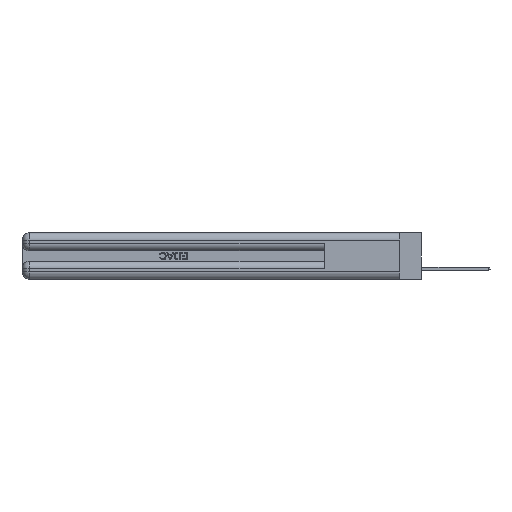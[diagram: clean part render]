
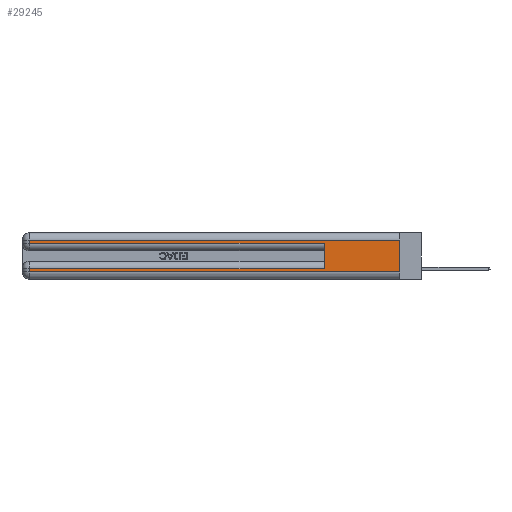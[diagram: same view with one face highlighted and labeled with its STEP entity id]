
A CAD part, left-side view. The second image highlights one B-rep face of the part: STEP entity #29245.
In plain terms, the highlighted planar face has unit normal (-1, 0, 0).
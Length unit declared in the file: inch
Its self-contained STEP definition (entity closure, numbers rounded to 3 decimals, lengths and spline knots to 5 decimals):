
#1138 = VECTOR ( 'NONE', #40566, 39.37008 ) ;
#1609 = CARTESIAN_POINT ( 'NONE',  ( 0., 0., 0.31 ) ) ;
#1885 = ORIENTED_EDGE ( 'NONE', *, *, #44636, .T. ) ;
#2199 = DIRECTION ( 'NONE',  ( 0., 0., 1. ) ) ;
#2629 = EDGE_CURVE ( 'NONE', #33854, #16843, #26381, .T. ) ;
#3667 = AXIS2_PLACEMENT_3D ( 'NONE', #36596, #48902, #10944 ) ;
#3835 = LINE ( 'NONE', #47116, #48518 ) ;
#3876 = CARTESIAN_POINT ( 'NONE',  ( 0., 2.94, 0.31 ) ) ;
#4954 = CARTESIAN_POINT ( 'NONE',  ( 0., 0., 0.085 ) ) ;
#5962 = DIRECTION ( 'NONE',  ( 0., 0., -1. ) ) ;
#7054 = CARTESIAN_POINT ( 'NONE',  ( 0., 0.6, 0.285 ) ) ;
#8005 = EDGE_LOOP ( 'NONE', ( #21062, #29447, #28083, #22457, #9642, #12252, #1885, #32867 ) ) ;
#8764 = DIRECTION ( 'NONE',  ( 0., 1., 0. ) ) ;
#9642 = ORIENTED_EDGE ( 'NONE', *, *, #23724, .F. ) ;
#9713 = CARTESIAN_POINT ( 'NONE',  ( 0., 0., 0.06 ) ) ;
#10944 = DIRECTION ( 'NONE',  ( 0., 0., -1. ) ) ;
#12252 = ORIENTED_EDGE ( 'NONE', *, *, #47221, .T. ) ;
#12604 = VERTEX_POINT ( 'NONE', #37717 ) ;
#12700 = CARTESIAN_POINT ( 'NONE',  ( 0., 2.94, 0.37 ) ) ;
#13351 = EDGE_CURVE ( 'NONE', #16843, #17796, #20602, .T. ) ;
#14908 = LINE ( 'NONE', #12700, #26865 ) ;
#15311 = VERTEX_POINT ( 'NONE', #33926 ) ;
#16782 = CARTESIAN_POINT ( 'NONE',  ( 0., 0., 0.37 ) ) ;
#16843 = VERTEX_POINT ( 'NONE', #41569 ) ;
#17676 = VECTOR ( 'NONE', #27738, 39.37008 ) ;
#17796 = VERTEX_POINT ( 'NONE', #7054 ) ;
#19616 = DIRECTION ( 'NONE',  ( 0., 0., -1. ) ) ;
#19625 = VERTEX_POINT ( 'NONE', #40451 ) ;
#20602 = LINE ( 'NONE', #23910, #17676 ) ;
#20718 = FACE_OUTER_BOUND ( 'NONE', #8005, .T. ) ;
#21062 = ORIENTED_EDGE ( 'NONE', *, *, #25597, .F. ) ;
#21465 = LINE ( 'NONE', #21615, #1138 ) ;
#21615 = CARTESIAN_POINT ( 'NONE',  ( 0., 0., 0.31 ) ) ;
#22457 = ORIENTED_EDGE ( 'NONE', *, *, #13351, .T. ) ;
#23704 = VERTEX_POINT ( 'NONE', #25021 ) ;
#23724 = EDGE_CURVE ( 'NONE', #19625, #17796, #3835, .T. ) ;
#23910 = CARTESIAN_POINT ( 'NONE',  ( 0., 0., 0.285 ) ) ;
#25021 = CARTESIAN_POINT ( 'NONE',  ( 0., 2.94, 0.06 ) ) ;
#25597 = EDGE_CURVE ( 'NONE', #44773, #12604, #28641, .T. ) ;
#25638 = VECTOR ( 'NONE', #5962, 39.37008 ) ;
#25729 = DIRECTION ( 'NONE',  ( 0., -1., 0. ) ) ;
#26381 = LINE ( 'NONE', #46326, #44881 ) ;
#26849 = VECTOR ( 'NONE', #8764, 39.37008 ) ;
#26865 = VECTOR ( 'NONE', #47048, 39.37008 ) ;
#27738 = DIRECTION ( 'NONE',  ( 0., -1., 0. ) ) ;
#28009 = LINE ( 'NONE', #4954, #26849 ) ;
#28083 = ORIENTED_EDGE ( 'NONE', *, *, #2629, .T. ) ;
#28641 = LINE ( 'NONE', #16782, #25638 ) ;
#29245 = ADVANCED_FACE ( 'NONE', ( #20718 ), #32581, .F. ) ;
#29447 = ORIENTED_EDGE ( 'NONE', *, *, #47834, .T. ) ;
#29568 = LINE ( 'NONE', #9713, #36084 ) ;
#32581 = PLANE ( 'NONE',  #3667 ) ;
#32867 = ORIENTED_EDGE ( 'NONE', *, *, #42263, .T. ) ;
#33854 = VERTEX_POINT ( 'NONE', #3876 ) ;
#33926 = CARTESIAN_POINT ( 'NONE',  ( 0., 2.94, 0.085 ) ) ;
#36084 = VECTOR ( 'NONE', #25729, 39.37008 ) ;
#36596 = CARTESIAN_POINT ( 'NONE',  ( 0., 0., 0.37 ) ) ;
#37717 = CARTESIAN_POINT ( 'NONE',  ( 0., 0., 0.06 ) ) ;
#40451 = CARTESIAN_POINT ( 'NONE',  ( 0., 0.6, 0.085 ) ) ;
#40566 = DIRECTION ( 'NONE',  ( 0., 1., 0. ) ) ;
#41569 = CARTESIAN_POINT ( 'NONE',  ( 0., 2.94, 0.285 ) ) ;
#42263 = EDGE_CURVE ( 'NONE', #23704, #12604, #29568, .T. ) ;
#44636 = EDGE_CURVE ( 'NONE', #15311, #23704, #14908, .T. ) ;
#44773 = VERTEX_POINT ( 'NONE', #1609 ) ;
#44881 = VECTOR ( 'NONE', #19616, 39.37008 ) ;
#46326 = CARTESIAN_POINT ( 'NONE',  ( 0., 2.94, 0.37 ) ) ;
#47048 = DIRECTION ( 'NONE',  ( 0., 0., -1. ) ) ;
#47116 = CARTESIAN_POINT ( 'NONE',  ( 0., 0.6, 0.145 ) ) ;
#47221 = EDGE_CURVE ( 'NONE', #19625, #15311, #28009, .T. ) ;
#47834 = EDGE_CURVE ( 'NONE', #44773, #33854, #21465, .T. ) ;
#48518 = VECTOR ( 'NONE', #2199, 39.37008 ) ;
#48902 = DIRECTION ( 'NONE',  ( 1., 0., 0. ) ) ;
